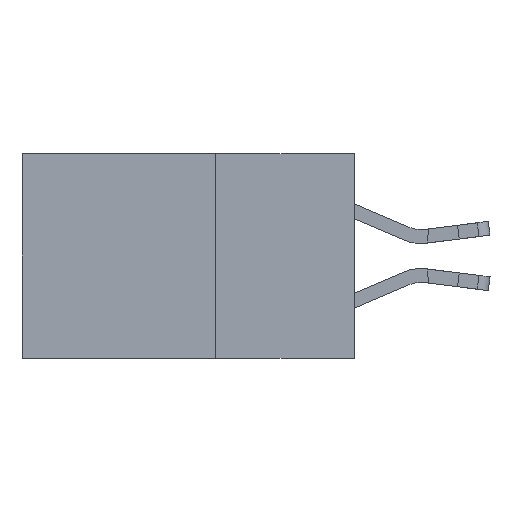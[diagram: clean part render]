
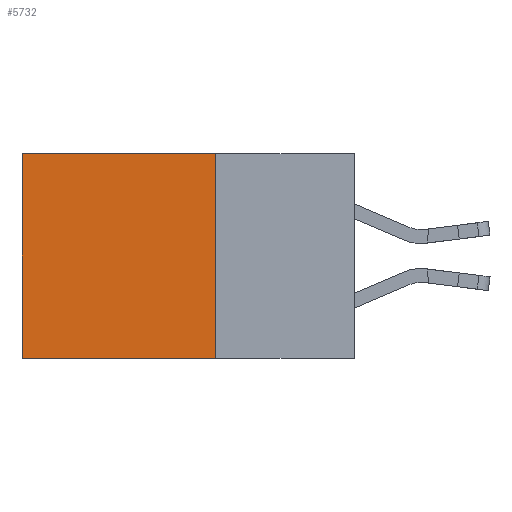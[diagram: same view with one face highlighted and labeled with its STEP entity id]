
A CAD part, left-side view. The second image highlights one B-rep face of the part: STEP entity #5732.
In plain terms, the highlighted planar face has unit normal (-1, 0, 0).
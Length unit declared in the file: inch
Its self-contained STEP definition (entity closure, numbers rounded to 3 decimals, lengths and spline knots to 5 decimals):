
#1225 = VECTOR ( 'NONE', #6225, 39.37008 ) ;
#2032 = VECTOR ( 'NONE', #6079, 39.37008 ) ;
#2748 = ORIENTED_EDGE ( 'NONE', *, *, #7682, .T. ) ;
#3147 = VERTEX_POINT ( 'NONE', #4012 ) ;
#3582 = VERTEX_POINT ( 'NONE', #13141 ) ;
#3787 = CARTESIAN_POINT ( 'NONE',  ( 0.298, 0.25, -0.37 ) ) ;
#4012 = CARTESIAN_POINT ( 'NONE',  ( 0.298, 0.25, -0.37 ) ) ;
#4174 = CARTESIAN_POINT ( 'NONE',  ( 0.298, 0.25, 0. ) ) ;
#4491 = CARTESIAN_POINT ( 'NONE',  ( 0.298, 0.25, 0. ) ) ;
#4807 = ORIENTED_EDGE ( 'NONE', *, *, #8188, .T. ) ;
#5232 = CARTESIAN_POINT ( 'NONE',  ( 0.298, 0.6, 0. ) ) ;
#5348 = LINE ( 'NONE', #3787, #2032 ) ;
#5732 = ADVANCED_FACE ( 'NONE', ( #14164 ), #7496, .F. ) ;
#6079 = DIRECTION ( 'NONE',  ( 0., 1., 0. ) ) ;
#6225 = DIRECTION ( 'NONE',  ( 0., 0., -1. ) ) ;
#7074 = LINE ( 'NONE', #4491, #10393 ) ;
#7274 = EDGE_CURVE ( 'NONE', #3147, #12390, #5348, .T. ) ;
#7496 = PLANE ( 'NONE',  #12596 ) ;
#7682 = EDGE_CURVE ( 'NONE', #11643, #3582, #7074, .T. ) ;
#8188 = EDGE_CURVE ( 'NONE', #3582, #12390, #13678, .T. ) ;
#8442 = CARTESIAN_POINT ( 'NONE',  ( 0.298, 0.6, -0.37 ) ) ;
#8638 = DIRECTION ( 'NONE',  ( 0., 0., -1. ) ) ;
#9470 = EDGE_CURVE ( 'NONE', #11643, #3147, #10574, .T. ) ;
#9851 = CARTESIAN_POINT ( 'NONE',  ( 0.298, 0.25, 0. ) ) ;
#10393 = VECTOR ( 'NONE', #13214, 39.37008 ) ;
#10574 = LINE ( 'NONE', #16031, #1225 ) ;
#11643 = VERTEX_POINT ( 'NONE', #4174 ) ;
#12172 = ORIENTED_EDGE ( 'NONE', *, *, #7274, .F. ) ;
#12251 = ORIENTED_EDGE ( 'NONE', *, *, #9470, .F. ) ;
#12347 = DIRECTION ( 'NONE',  ( 1., 0., 0. ) ) ;
#12390 = VERTEX_POINT ( 'NONE', #8442 ) ;
#12596 = AXIS2_PLACEMENT_3D ( 'NONE', #9851, #12347, #8638 ) ;
#12638 = DIRECTION ( 'NONE',  ( 0., 0., -1. ) ) ;
#12724 = VECTOR ( 'NONE', #12638, 39.37008 ) ;
#13141 = CARTESIAN_POINT ( 'NONE',  ( 0.298, 0.6, 0. ) ) ;
#13214 = DIRECTION ( 'NONE',  ( 0., 1., 0. ) ) ;
#13678 = LINE ( 'NONE', #5232, #12724 ) ;
#14088 = EDGE_LOOP ( 'NONE', ( #4807, #12172, #12251, #2748 ) ) ;
#14164 = FACE_OUTER_BOUND ( 'NONE', #14088, .T. ) ;
#16031 = CARTESIAN_POINT ( 'NONE',  ( 0.298, 0.25, 0. ) ) ;
